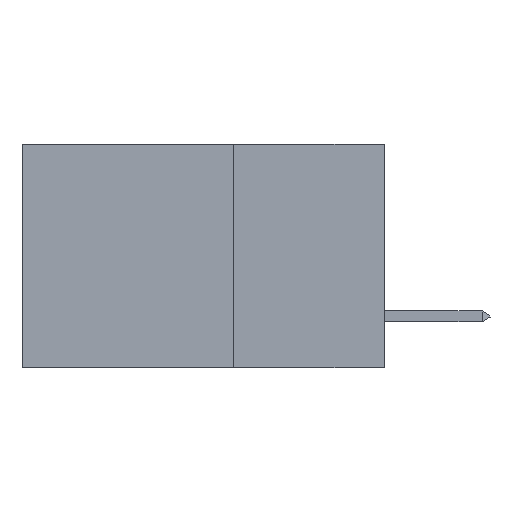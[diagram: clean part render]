
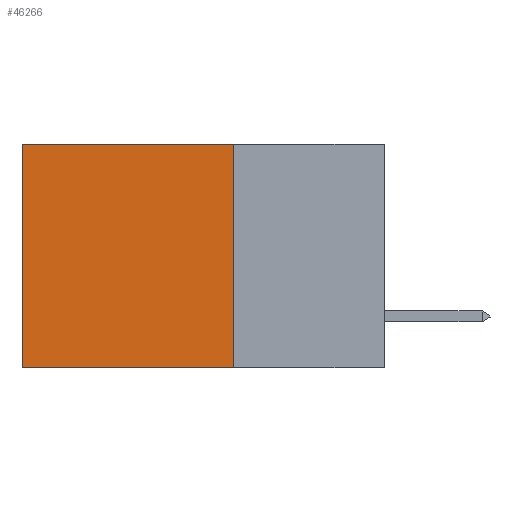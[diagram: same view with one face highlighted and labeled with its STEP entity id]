
A CAD part, left-side view. The second image highlights one B-rep face of the part: STEP entity #46266.
In plain terms, the highlighted planar face has unit normal (-1, 0, 0).
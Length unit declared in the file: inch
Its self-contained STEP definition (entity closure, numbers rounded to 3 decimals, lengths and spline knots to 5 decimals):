
#1189 = VERTEX_POINT ( 'NONE', #43792 ) ;
#1515 = PLANE ( 'NONE',  #9169 ) ;
#2883 = DIRECTION ( 'NONE',  ( 0., 1., 0. ) ) ;
#3119 = ORIENTED_EDGE ( 'NONE', *, *, #12895, .F. ) ;
#4848 = DIRECTION ( 'NONE',  ( 0., 0., -1. ) ) ;
#5946 = FACE_OUTER_BOUND ( 'NONE', #25758, .T. ) ;
#6075 = CARTESIAN_POINT ( 'NONE',  ( 0.2875, 0.6, 0. ) ) ;
#6304 = DIRECTION ( 'NONE',  ( 0., 1., 0. ) ) ;
#9169 = AXIS2_PLACEMENT_3D ( 'NONE', #26597, #30745, #4848 ) ;
#9678 = EDGE_CURVE ( 'NONE', #11438, #43577, #18502, .T. ) ;
#9900 = LINE ( 'NONE', #17115, #41195 ) ;
#10032 = LINE ( 'NONE', #31706, #25318 ) ;
#11438 = VERTEX_POINT ( 'NONE', #37751 ) ;
#12895 = EDGE_CURVE ( 'NONE', #11438, #1189, #10032, .T. ) ;
#13475 = DIRECTION ( 'NONE',  ( 0., 0., -1. ) ) ;
#14221 = LINE ( 'NONE', #6075, #16452 ) ;
#14750 = EDGE_CURVE ( 'NONE', #1189, #44794, #9900, .T. ) ;
#15650 = ORIENTED_EDGE ( 'NONE', *, *, #14750, .F. ) ;
#15658 = VECTOR ( 'NONE', #2883, 39.37008 ) ;
#16452 = VECTOR ( 'NONE', #27340, 39.37008 ) ;
#17115 = CARTESIAN_POINT ( 'NONE',  ( 0.2875, 0.25, -0.37 ) ) ;
#17573 = EDGE_CURVE ( 'NONE', #43577, #44794, #14221, .T. ) ;
#18502 = LINE ( 'NONE', #32434, #15658 ) ;
#25318 = VECTOR ( 'NONE', #13475, 39.37008 ) ;
#25758 = EDGE_LOOP ( 'NONE', ( #40014, #15650, #3119, #43429 ) ) ;
#26597 = CARTESIAN_POINT ( 'NONE',  ( 0.2875, 0.25, 0. ) ) ;
#27340 = DIRECTION ( 'NONE',  ( 0., 0., -1. ) ) ;
#30745 = DIRECTION ( 'NONE',  ( 1., 0., 0. ) ) ;
#31706 = CARTESIAN_POINT ( 'NONE',  ( 0.2875, 0.25, 0. ) ) ;
#31877 = CARTESIAN_POINT ( 'NONE',  ( 0.2875, 0.6, 0. ) ) ;
#32434 = CARTESIAN_POINT ( 'NONE',  ( 0.2875, 0.25, 0. ) ) ;
#37751 = CARTESIAN_POINT ( 'NONE',  ( 0.2875, 0.25, 0. ) ) ;
#40014 = ORIENTED_EDGE ( 'NONE', *, *, #17573, .T. ) ;
#41195 = VECTOR ( 'NONE', #6304, 39.37008 ) ;
#43429 = ORIENTED_EDGE ( 'NONE', *, *, #9678, .T. ) ;
#43577 = VERTEX_POINT ( 'NONE', #31877 ) ;
#43792 = CARTESIAN_POINT ( 'NONE',  ( 0.2875, 0.25, -0.37 ) ) ;
#44794 = VERTEX_POINT ( 'NONE', #46378 ) ;
#46266 = ADVANCED_FACE ( 'NONE', ( #5946 ), #1515, .F. ) ;
#46378 = CARTESIAN_POINT ( 'NONE',  ( 0.2875, 0.6, -0.37 ) ) ;
